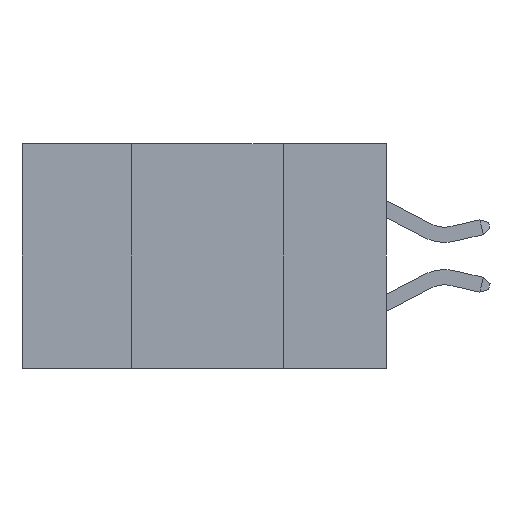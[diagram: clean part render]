
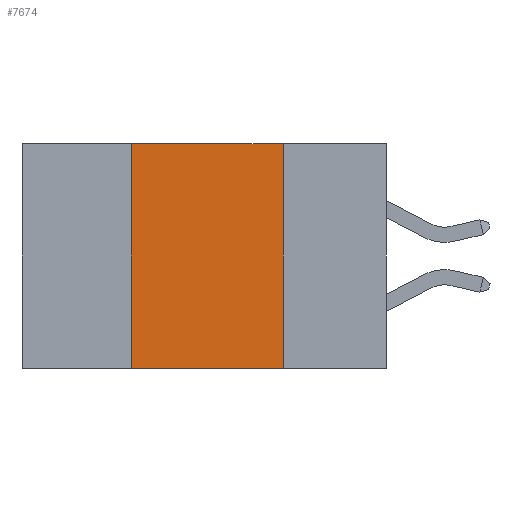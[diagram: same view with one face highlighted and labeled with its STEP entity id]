
A CAD part, left-side view. The second image highlights one B-rep face of the part: STEP entity #7674.
In plain terms, the highlighted planar face has unit normal (-1, 0, 0).
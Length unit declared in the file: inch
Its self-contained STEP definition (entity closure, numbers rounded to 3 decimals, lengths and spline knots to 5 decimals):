
#162 = VERTEX_POINT ( 'NONE', #3548 ) ;
#696 = VECTOR ( 'NONE', #8041, 39.37008 ) ;
#1169 = FACE_OUTER_BOUND ( 'NONE', #14701, .T. ) ;
#1437 = EDGE_CURVE ( 'NONE', #7665, #8063, #10029, .T. ) ;
#2319 = CARTESIAN_POINT ( 'NONE',  ( 0., 0.42, 0. ) ) ;
#2653 = VERTEX_POINT ( 'NONE', #8755 ) ;
#2764 = CARTESIAN_POINT ( 'NONE',  ( 0., 0.6, 0. ) ) ;
#2895 = DIRECTION ( 'NONE',  ( 0., 0., -1. ) ) ;
#3158 = LINE ( 'NONE', #6844, #696 ) ;
#3548 = CARTESIAN_POINT ( 'NONE',  ( 0., 0.42, -0.37 ) ) ;
#4122 = ORIENTED_EDGE ( 'NONE', *, *, #9344, .T. ) ;
#4157 = AXIS2_PLACEMENT_3D ( 'NONE', #2764, #7228, #2895 ) ;
#5335 = ORIENTED_EDGE ( 'NONE', *, *, #8603, .F. ) ;
#5394 = CARTESIAN_POINT ( 'NONE',  ( 0., 0.17, 0. ) ) ;
#5974 = VECTOR ( 'NONE', #13017, 39.37008 ) ;
#6071 = ORIENTED_EDGE ( 'NONE', *, *, #14340, .F. ) ;
#6557 = CARTESIAN_POINT ( 'NONE',  ( 0., 0.42, 0. ) ) ;
#6844 = CARTESIAN_POINT ( 'NONE',  ( 0., 0.6, -0.37 ) ) ;
#7228 = DIRECTION ( 'NONE',  ( 1., 0., 0. ) ) ;
#7665 = VERTEX_POINT ( 'NONE', #2319 ) ;
#7674 = ADVANCED_FACE ( 'NONE', ( #1169 ), #11039, .F. ) ;
#7995 = DIRECTION ( 'NONE',  ( 0., 0., 1. ) ) ;
#8041 = DIRECTION ( 'NONE',  ( 0., -1., 0. ) ) ;
#8063 = VERTEX_POINT ( 'NONE', #5394 ) ;
#8603 = EDGE_CURVE ( 'NONE', #8063, #2653, #9464, .T. ) ;
#8610 = CARTESIAN_POINT ( 'NONE',  ( 0., 0.17, 0. ) ) ;
#8755 = CARTESIAN_POINT ( 'NONE',  ( 0., 0.17, -0.37 ) ) ;
#9344 = EDGE_CURVE ( 'NONE', #162, #2653, #3158, .T. ) ;
#9464 = LINE ( 'NONE', #8610, #9911 ) ;
#9911 = VECTOR ( 'NONE', #11610, 39.37008 ) ;
#10029 = LINE ( 'NONE', #11497, #5974 ) ;
#10861 = ORIENTED_EDGE ( 'NONE', *, *, #1437, .F. ) ;
#11039 = PLANE ( 'NONE',  #4157 ) ;
#11497 = CARTESIAN_POINT ( 'NONE',  ( 0., 0.6, 0. ) ) ;
#11610 = DIRECTION ( 'NONE',  ( 0., 0., -1. ) ) ;
#12747 = LINE ( 'NONE', #6557, #18430 ) ;
#13017 = DIRECTION ( 'NONE',  ( 0., -1., 0. ) ) ;
#14340 = EDGE_CURVE ( 'NONE', #162, #7665, #12747, .T. ) ;
#14701 = EDGE_LOOP ( 'NONE', ( #5335, #10861, #6071, #4122 ) ) ;
#18430 = VECTOR ( 'NONE', #7995, 39.37008 ) ;
